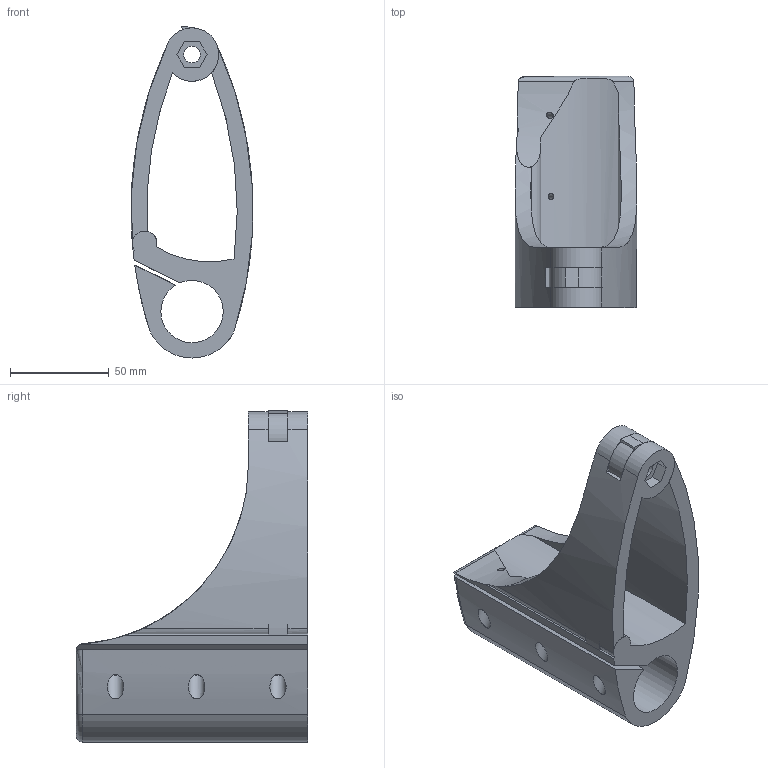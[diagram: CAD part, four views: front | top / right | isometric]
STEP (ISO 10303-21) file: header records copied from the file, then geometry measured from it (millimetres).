
FILE_DESCRIPTION(/* description */ (''),/* implementation_level */ '2;1');
FILE_NAME(/* name */ 'Tailhook-Mod-2.step',/* time_stamp */ '2018-01-00T00:00:00-01:00',/* author */ ('fosscadbot'),/* organization */ ('fosscad'),/* preprocessor_version */ 'ST-DEVELOPER v17',/* originating_system */ 'Autodesk Translation Framework v7.1.0.215',/* authorisation */ '');
FILE_SCHEMA (('AUTOMOTIVE_DESIGN { 1 0 10303 214 3 1 1 }'));
Length unit declared in the file: millimetre
Products named in the file (3): Tailhook-Mod-2; Component1; Component2
Assembly tree (2 placements, depth 2):
  Tailhook-Mod-2
    Component1
    Component2
Bounding box: 61.69 x 117 x 167.95 mm (x, y, z)
Volume: 267159.6 mm3; surface area: 72010.7 mm2
Topology: 2 solids, 2 shells, 77 faces, 195 edges, 126 vertices
Faces by surface type: cylinder 40, plane 34, torus 3
Full cylindrical faces by diameter (mm): 3 x6, 8.2 x3, 8.5 x3
Entity records: 2830 total; most frequent: CARTESIAN_POINT 831, DIRECTION 408, ORIENTED_EDGE 392, EDGE_CURVE 196, AXIS2_PLACEMENT_3D 156, VERTEX_POINT 126, EDGE_LOOP 99, LINE 96
